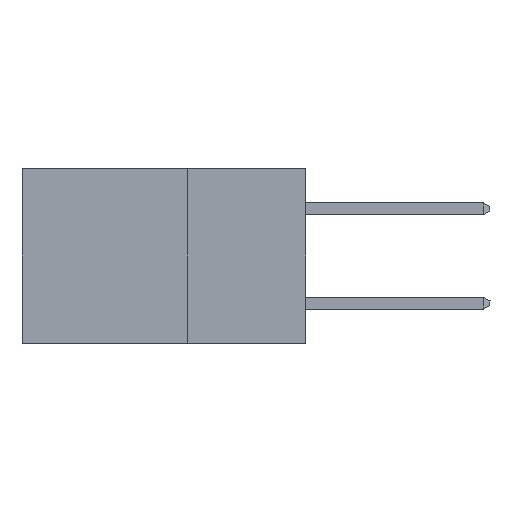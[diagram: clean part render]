
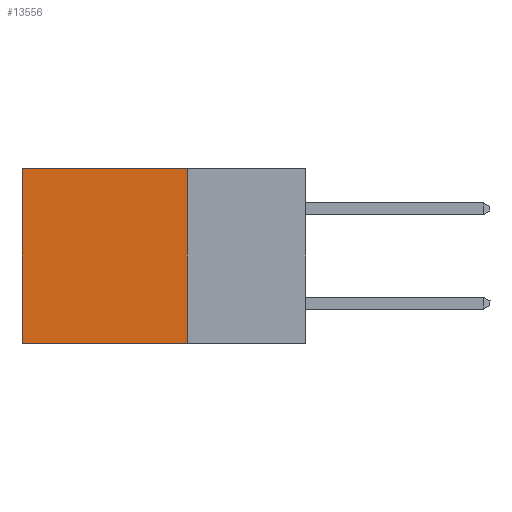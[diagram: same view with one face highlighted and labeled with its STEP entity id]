
A CAD part, left-side view. The second image highlights one B-rep face of the part: STEP entity #13556.
In plain terms, the highlighted planar face has unit normal (-1, 0, 0).
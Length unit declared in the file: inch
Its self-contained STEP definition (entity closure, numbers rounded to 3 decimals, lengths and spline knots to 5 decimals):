
#248 = CARTESIAN_POINT ( 'NONE',  ( 0.298, 0.25, 0. ) ) ;
#254 = ORIENTED_EDGE ( 'NONE', *, *, #5265, .F. ) ;
#602 = DIRECTION ( 'NONE',  ( 0., 1., 0. ) ) ;
#671 = VECTOR ( 'NONE', #13202, 39.37008 ) ;
#675 = CARTESIAN_POINT ( 'NONE',  ( 0.298, 0.6, 0. ) ) ;
#1460 = DIRECTION ( 'NONE',  ( 0., 1., 0. ) ) ;
#1517 = CARTESIAN_POINT ( 'NONE',  ( 0.298, 0.25, 0. ) ) ;
#2013 = DIRECTION ( 'NONE',  ( 0., 0., -1. ) ) ;
#2032 = LINE ( 'NONE', #6331, #671 ) ;
#2246 = EDGE_CURVE ( 'NONE', #13357, #12810, #12753, .T. ) ;
#2496 = CARTESIAN_POINT ( 'NONE',  ( 0.298, 0.6, -0.37 ) ) ;
#2718 = EDGE_CURVE ( 'NONE', #12810, #10446, #2032, .T. ) ;
#3471 = EDGE_LOOP ( 'NONE', ( #11007, #6748, #254, #4955 ) ) ;
#3731 = CARTESIAN_POINT ( 'NONE',  ( 0.298, 0.25, -0.37 ) ) ;
#3805 = EDGE_CURVE ( 'NONE', #14267, #10446, #9513, .T. ) ;
#4045 = DIRECTION ( 'NONE',  ( 0., 0., -1. ) ) ;
#4198 = CARTESIAN_POINT ( 'NONE',  ( 0.298, 0.25, 0. ) ) ;
#4955 = ORIENTED_EDGE ( 'NONE', *, *, #2246, .T. ) ;
#5265 = EDGE_CURVE ( 'NONE', #13357, #14267, #10573, .T. ) ;
#5831 = VECTOR ( 'NONE', #602, 39.37008 ) ;
#6331 = CARTESIAN_POINT ( 'NONE',  ( 0.298, 0.6, 0. ) ) ;
#6748 = ORIENTED_EDGE ( 'NONE', *, *, #3805, .F. ) ;
#7118 = VECTOR ( 'NONE', #1460, 39.37008 ) ;
#7247 = VECTOR ( 'NONE', #4045, 39.37008 ) ;
#8688 = DIRECTION ( 'NONE',  ( 1., 0., 0. ) ) ;
#9513 = LINE ( 'NONE', #11796, #5831 ) ;
#10446 = VERTEX_POINT ( 'NONE', #2496 ) ;
#10573 = LINE ( 'NONE', #11872, #7247 ) ;
#11007 = ORIENTED_EDGE ( 'NONE', *, *, #2718, .T. ) ;
#11796 = CARTESIAN_POINT ( 'NONE',  ( 0.298, 0.25, -0.37 ) ) ;
#11872 = CARTESIAN_POINT ( 'NONE',  ( 0.298, 0.25, 0. ) ) ;
#11941 = PLANE ( 'NONE',  #13094 ) ;
#12578 = FACE_OUTER_BOUND ( 'NONE', #3471, .T. ) ;
#12753 = LINE ( 'NONE', #248, #7118 ) ;
#12810 = VERTEX_POINT ( 'NONE', #675 ) ;
#13094 = AXIS2_PLACEMENT_3D ( 'NONE', #4198, #8688, #2013 ) ;
#13202 = DIRECTION ( 'NONE',  ( 0., 0., -1. ) ) ;
#13357 = VERTEX_POINT ( 'NONE', #1517 ) ;
#13556 = ADVANCED_FACE ( 'NONE', ( #12578 ), #11941, .F. ) ;
#14267 = VERTEX_POINT ( 'NONE', #3731 ) ;
